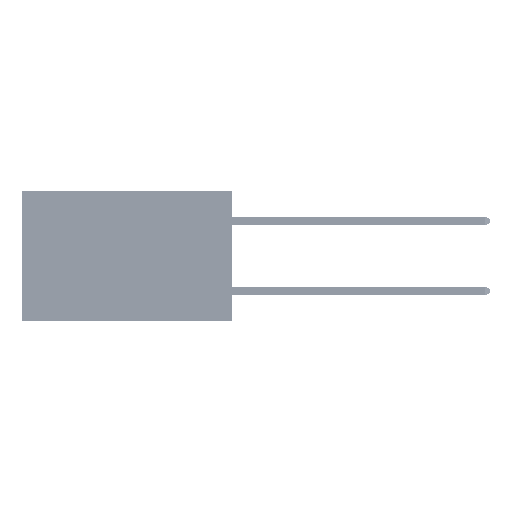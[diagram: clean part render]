
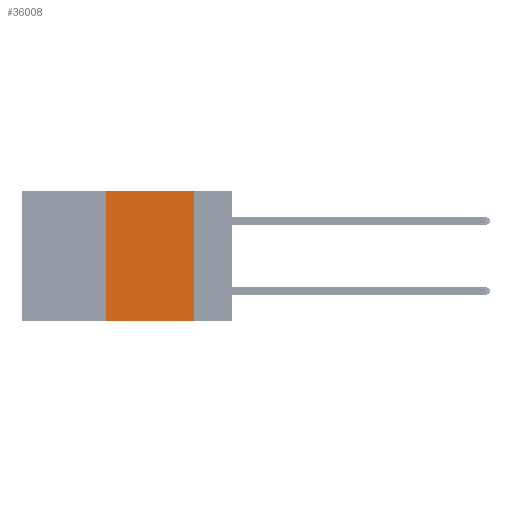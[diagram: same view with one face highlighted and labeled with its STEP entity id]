
A CAD part, left-side view. The second image highlights one B-rep face of the part: STEP entity #36008.
In plain terms, the highlighted planar face has unit normal (-1, 0, 0).
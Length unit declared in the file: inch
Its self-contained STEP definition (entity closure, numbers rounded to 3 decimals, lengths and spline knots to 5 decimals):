
#4748 = DIRECTION ( 'NONE',  ( 1., 0., 0. ) ) ;
#5476 = VERTEX_POINT ( 'NONE', #34704 ) ;
#6400 = ORIENTED_EDGE ( 'NONE', *, *, #12302, .F. ) ;
#7122 = LINE ( 'NONE', #43177, #47416 ) ;
#8380 = ORIENTED_EDGE ( 'NONE', *, *, #20222, .F. ) ;
#9087 = VECTOR ( 'NONE', #33962, 39.37008 ) ;
#9910 = ORIENTED_EDGE ( 'NONE', *, *, #31761, .T. ) ;
#10590 = CARTESIAN_POINT ( 'NONE',  ( 0., 0.11, 0. ) ) ;
#11783 = CARTESIAN_POINT ( 'NONE',  ( 0., 0.11, -0.37 ) ) ;
#12302 = EDGE_CURVE ( 'NONE', #49593, #27528, #7122, .T. ) ;
#13441 = ORIENTED_EDGE ( 'NONE', *, *, #50902, .F. ) ;
#18534 = CARTESIAN_POINT ( 'NONE',  ( 0., 0.6, -0.37 ) ) ;
#18777 = AXIS2_PLACEMENT_3D ( 'NONE', #36060, #4748, #28623 ) ;
#19582 = DIRECTION ( 'NONE',  ( 0., 0., -1. ) ) ;
#20222 = EDGE_CURVE ( 'NONE', #32541, #5476, #28280, .T. ) ;
#20494 = VECTOR ( 'NONE', #22695, 39.37008 ) ;
#20757 = EDGE_LOOP ( 'NONE', ( #6400, #13441, #8380, #9910 ) ) ;
#22695 = DIRECTION ( 'NONE',  ( 0., -1., 0. ) ) ;
#22988 = LINE ( 'NONE', #18534, #20494 ) ;
#23533 = CARTESIAN_POINT ( 'NONE',  ( 0., 0.36, 0. ) ) ;
#27528 = VERTEX_POINT ( 'NONE', #11783 ) ;
#28280 = LINE ( 'NONE', #23533, #49413 ) ;
#28623 = DIRECTION ( 'NONE',  ( 0., 0., -1. ) ) ;
#31485 = DIRECTION ( 'NONE',  ( 0., 0., 1. ) ) ;
#31761 = EDGE_CURVE ( 'NONE', #32541, #27528, #22988, .T. ) ;
#32541 = VERTEX_POINT ( 'NONE', #50866 ) ;
#33962 = DIRECTION ( 'NONE',  ( 0., -1., 0. ) ) ;
#34070 = FACE_OUTER_BOUND ( 'NONE', #20757, .T. ) ;
#34704 = CARTESIAN_POINT ( 'NONE',  ( 0., 0.36, 0. ) ) ;
#36008 = ADVANCED_FACE ( 'NONE', ( #34070 ), #48207, .F. ) ;
#36060 = CARTESIAN_POINT ( 'NONE',  ( 0., 0.6, 0. ) ) ;
#43177 = CARTESIAN_POINT ( 'NONE',  ( 0., 0.11, 0. ) ) ;
#46940 = LINE ( 'NONE', #50266, #9087 ) ;
#47416 = VECTOR ( 'NONE', #19582, 39.37008 ) ;
#48207 = PLANE ( 'NONE',  #18777 ) ;
#49413 = VECTOR ( 'NONE', #31485, 39.37008 ) ;
#49593 = VERTEX_POINT ( 'NONE', #10590 ) ;
#50266 = CARTESIAN_POINT ( 'NONE',  ( 0., 0.6, 0. ) ) ;
#50866 = CARTESIAN_POINT ( 'NONE',  ( 0., 0.36, -0.37 ) ) ;
#50902 = EDGE_CURVE ( 'NONE', #5476, #49593, #46940, .T. ) ;
